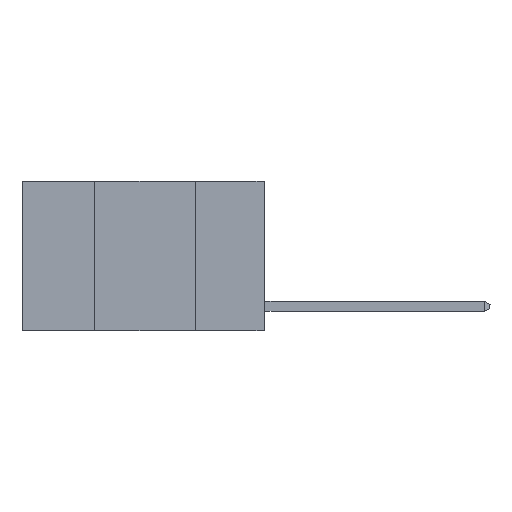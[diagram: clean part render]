
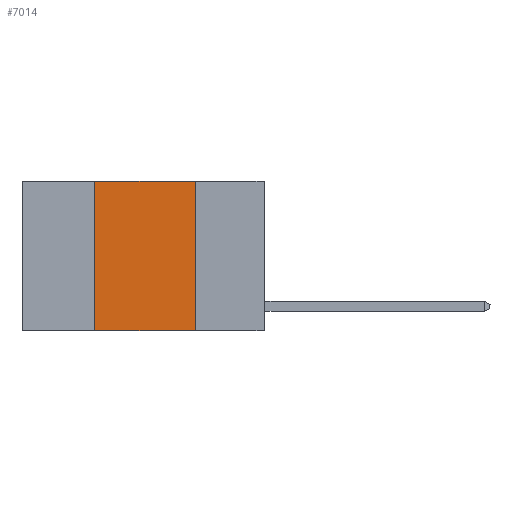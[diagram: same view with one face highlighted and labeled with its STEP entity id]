
A CAD part, left-side view. The second image highlights one B-rep face of the part: STEP entity #7014.
In plain terms, the highlighted planar face has unit normal (-1, 0, 0).
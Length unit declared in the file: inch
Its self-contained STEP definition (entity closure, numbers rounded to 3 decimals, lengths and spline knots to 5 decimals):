
#54 = EDGE_CURVE ( 'NONE', #9599, #17261, #2248, .T. ) ;
#921 = CARTESIAN_POINT ( 'NONE',  ( 0., 0.6, -0.37 ) ) ;
#1469 = DIRECTION ( 'NONE',  ( 0., 0., -1. ) ) ;
#2047 = EDGE_CURVE ( 'NONE', #2459, #9599, #5307, .T. ) ;
#2248 = LINE ( 'NONE', #15773, #9714 ) ;
#2323 = EDGE_CURVE ( 'NONE', #6749, #2459, #18166, .T. ) ;
#2459 = VERTEX_POINT ( 'NONE', #8230 ) ;
#2971 = CARTESIAN_POINT ( 'NONE',  ( 0., 0.42, -0.37 ) ) ;
#4990 = CARTESIAN_POINT ( 'NONE',  ( 0., 0.6, 0. ) ) ;
#5185 = CARTESIAN_POINT ( 'NONE',  ( 0., 0.42, 0. ) ) ;
#5307 = LINE ( 'NONE', #12623, #12269 ) ;
#5491 = CARTESIAN_POINT ( 'NONE',  ( 0., 0.17, 0. ) ) ;
#6398 = DIRECTION ( 'NONE',  ( 1., 0., 0. ) ) ;
#6584 = DIRECTION ( 'NONE',  ( 0., 0., 1. ) ) ;
#6652 = EDGE_LOOP ( 'NONE', ( #8039, #6723, #17427, #13271 ) ) ;
#6723 = ORIENTED_EDGE ( 'NONE', *, *, #2047, .F. ) ;
#6749 = VERTEX_POINT ( 'NONE', #2971 ) ;
#7014 = ADVANCED_FACE ( 'NONE', ( #10464 ), #13349, .F. ) ;
#7027 = VECTOR ( 'NONE', #6584, 39.37008 ) ;
#8039 = ORIENTED_EDGE ( 'NONE', *, *, #54, .F. ) ;
#8230 = CARTESIAN_POINT ( 'NONE',  ( 0., 0.42, 0. ) ) ;
#9119 = AXIS2_PLACEMENT_3D ( 'NONE', #4990, #6398, #16169 ) ;
#9296 = DIRECTION ( 'NONE',  ( 0., -1., 0. ) ) ;
#9599 = VERTEX_POINT ( 'NONE', #5491 ) ;
#9714 = VECTOR ( 'NONE', #1469, 39.37008 ) ;
#10081 = VECTOR ( 'NONE', #9296, 39.37008 ) ;
#10150 = EDGE_CURVE ( 'NONE', #6749, #17261, #13842, .T. ) ;
#10464 = FACE_OUTER_BOUND ( 'NONE', #6652, .T. ) ;
#12269 = VECTOR ( 'NONE', #14052, 39.37008 ) ;
#12623 = CARTESIAN_POINT ( 'NONE',  ( 0., 0.6, 0. ) ) ;
#13271 = ORIENTED_EDGE ( 'NONE', *, *, #10150, .T. ) ;
#13349 = PLANE ( 'NONE',  #9119 ) ;
#13842 = LINE ( 'NONE', #921, #10081 ) ;
#13906 = CARTESIAN_POINT ( 'NONE',  ( 0., 0.17, -0.37 ) ) ;
#14052 = DIRECTION ( 'NONE',  ( 0., -1., 0. ) ) ;
#15773 = CARTESIAN_POINT ( 'NONE',  ( 0., 0.17, 0. ) ) ;
#16169 = DIRECTION ( 'NONE',  ( 0., 0., -1. ) ) ;
#17261 = VERTEX_POINT ( 'NONE', #13906 ) ;
#17427 = ORIENTED_EDGE ( 'NONE', *, *, #2323, .F. ) ;
#18166 = LINE ( 'NONE', #5185, #7027 ) ;
